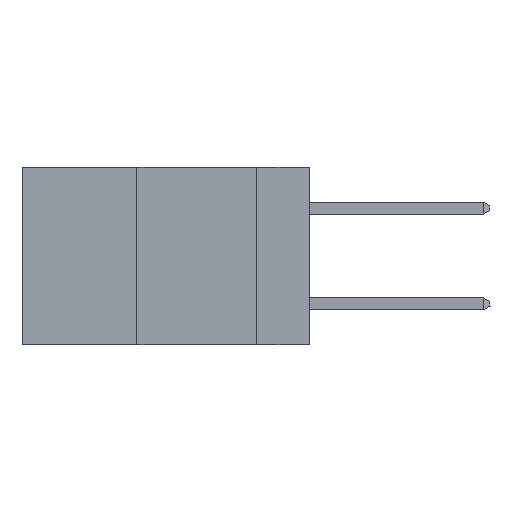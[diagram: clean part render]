
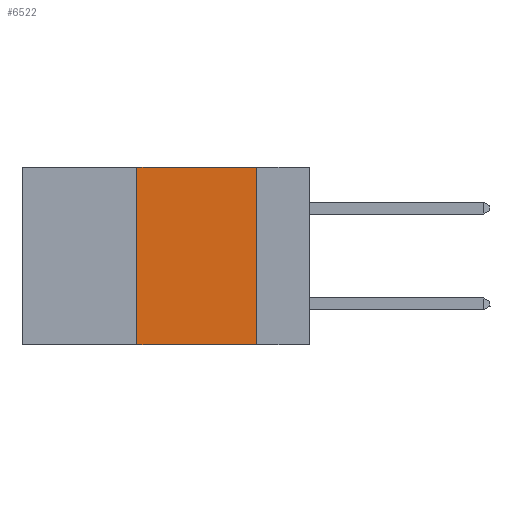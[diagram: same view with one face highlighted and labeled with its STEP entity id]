
A CAD part, left-side view. The second image highlights one B-rep face of the part: STEP entity #6522.
In plain terms, the highlighted planar face has unit normal (-1, 0, 0).
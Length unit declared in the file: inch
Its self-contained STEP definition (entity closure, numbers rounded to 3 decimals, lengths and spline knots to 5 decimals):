
#1871 = LINE ( 'NONE', #2376, #23234 ) ;
#2376 = CARTESIAN_POINT ( 'NONE',  ( 0., 0.6, 0. ) ) ;
#2874 = DIRECTION ( 'NONE',  ( 0., -1., 0. ) ) ;
#3856 = EDGE_CURVE ( 'NONE', #14840, #23698, #1871, .T. ) ;
#3948 = CARTESIAN_POINT ( 'NONE',  ( 0., 0.6, 0. ) ) ;
#4453 = CARTESIAN_POINT ( 'NONE',  ( 0., 0.11, -0.37 ) ) ;
#4501 = DIRECTION ( 'NONE',  ( 0., 0., 1. ) ) ;
#5582 = AXIS2_PLACEMENT_3D ( 'NONE', #3948, #13332, #29237 ) ;
#6522 = ADVANCED_FACE ( 'NONE', ( #9347 ), #20080, .F. ) ;
#8312 = ORIENTED_EDGE ( 'NONE', *, *, #23407, .F. ) ;
#9339 = VECTOR ( 'NONE', #4501, 39.37008 ) ;
#9347 = FACE_OUTER_BOUND ( 'NONE', #21023, .T. ) ;
#9875 = EDGE_CURVE ( 'NONE', #23149, #20748, #26594, .T. ) ;
#10146 = CARTESIAN_POINT ( 'NONE',  ( 0., 0.11, 0. ) ) ;
#10519 = VECTOR ( 'NONE', #21179, 39.37008 ) ;
#11042 = DIRECTION ( 'NONE',  ( 0., -1., 0. ) ) ;
#11927 = CARTESIAN_POINT ( 'NONE',  ( 0., 0.11, 0. ) ) ;
#13332 = DIRECTION ( 'NONE',  ( 1., 0., 0. ) ) ;
#14709 = EDGE_CURVE ( 'NONE', #23149, #14840, #26277, .T. ) ;
#14840 = VERTEX_POINT ( 'NONE', #23347 ) ;
#18076 = CARTESIAN_POINT ( 'NONE',  ( 0., 0.6, -0.37 ) ) ;
#18584 = CARTESIAN_POINT ( 'NONE',  ( 0., 0.36, -0.37 ) ) ;
#18667 = ORIENTED_EDGE ( 'NONE', *, *, #14709, .F. ) ;
#19917 = CARTESIAN_POINT ( 'NONE',  ( 0., 0.36, 0. ) ) ;
#20080 = PLANE ( 'NONE',  #5582 ) ;
#20748 = VERTEX_POINT ( 'NONE', #4453 ) ;
#21023 = EDGE_LOOP ( 'NONE', ( #8312, #22550, #18667, #25595 ) ) ;
#21179 = DIRECTION ( 'NONE',  ( 0., 0., -1. ) ) ;
#22550 = ORIENTED_EDGE ( 'NONE', *, *, #3856, .F. ) ;
#23149 = VERTEX_POINT ( 'NONE', #18584 ) ;
#23234 = VECTOR ( 'NONE', #2874, 39.37008 ) ;
#23347 = CARTESIAN_POINT ( 'NONE',  ( 0., 0.36, 0. ) ) ;
#23407 = EDGE_CURVE ( 'NONE', #23698, #20748, #29266, .T. ) ;
#23698 = VERTEX_POINT ( 'NONE', #10146 ) ;
#25595 = ORIENTED_EDGE ( 'NONE', *, *, #9875, .T. ) ;
#25874 = VECTOR ( 'NONE', #11042, 39.37008 ) ;
#26277 = LINE ( 'NONE', #19917, #9339 ) ;
#26594 = LINE ( 'NONE', #18076, #25874 ) ;
#29237 = DIRECTION ( 'NONE',  ( 0., 0., -1. ) ) ;
#29266 = LINE ( 'NONE', #11927, #10519 ) ;
